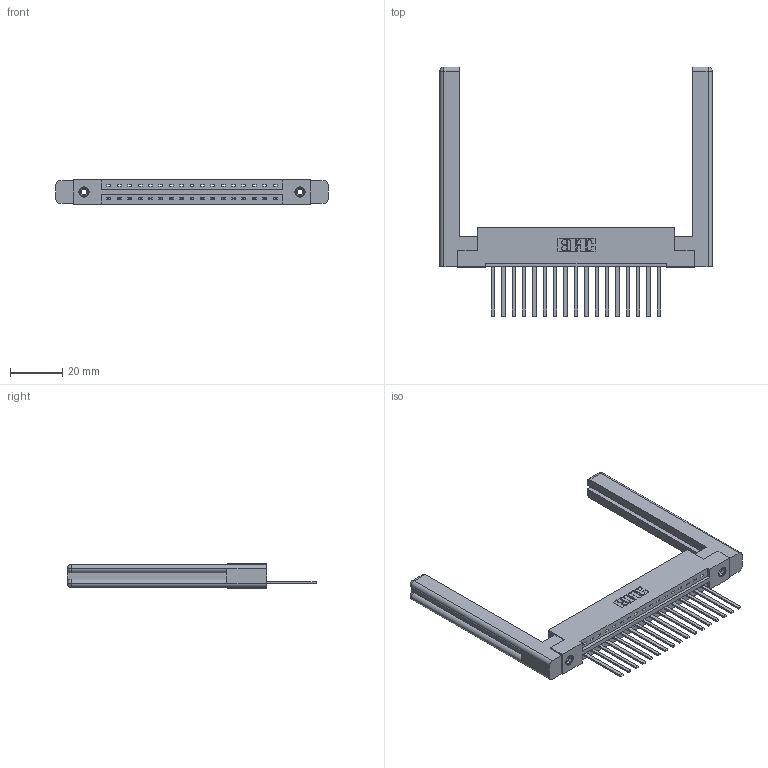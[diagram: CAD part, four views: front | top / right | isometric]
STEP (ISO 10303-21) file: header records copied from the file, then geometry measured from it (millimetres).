
FILE_DESCRIPTION (( 'STEP AP203' ), '1' );
FILE_NAME ('337-017-544-158.STEP', '2019-09-28T19:14:07', ( '' ), ( '' ), 'SwSTEP 2.0', 'SolidWorks 2016', '' );
FILE_SCHEMA (( 'CONFIG_CONTROL_DESIGN' ));
Length unit declared in the file: inch
Products named in the file (5): 307-220-058; 345-250-001_345-250-001-102; 337-017-544-158; 337 Part_Flush Mounting Lugs - 0.156 Dia-TI; 345-292-001_345-293-144
Assembly tree (22 placements, depth 2):
  337-017-544-158
    337 Part_Flush Mounting Lugs - 0.156 Dia-TI
    345-292-001_345-293-144  x17
    345-250-001_345-250-001-102  x2
    307-220-058  x2
Bounding box: 103.99 x 95.38 x 9.4 mm (x, y, z)
Volume: 17854 mm3; surface area: 16770.3 mm2
Topology: 22 solids, 22 shells, 1208 faces, 3555 edges, 2334 vertices
Faces by surface type: plane 868, cylinder 316, cone 12, torus 12
Entity records: 18320 total; most frequent: CARTESIAN_POINT 3188, ORIENTED_EDGE 3080, DIRECTION 2750, EDGE_CURVE 1540, LINE 1368, VECTOR 1368, VERTEX_POINT 1018, AXIS2_PLACEMENT_3D 691
